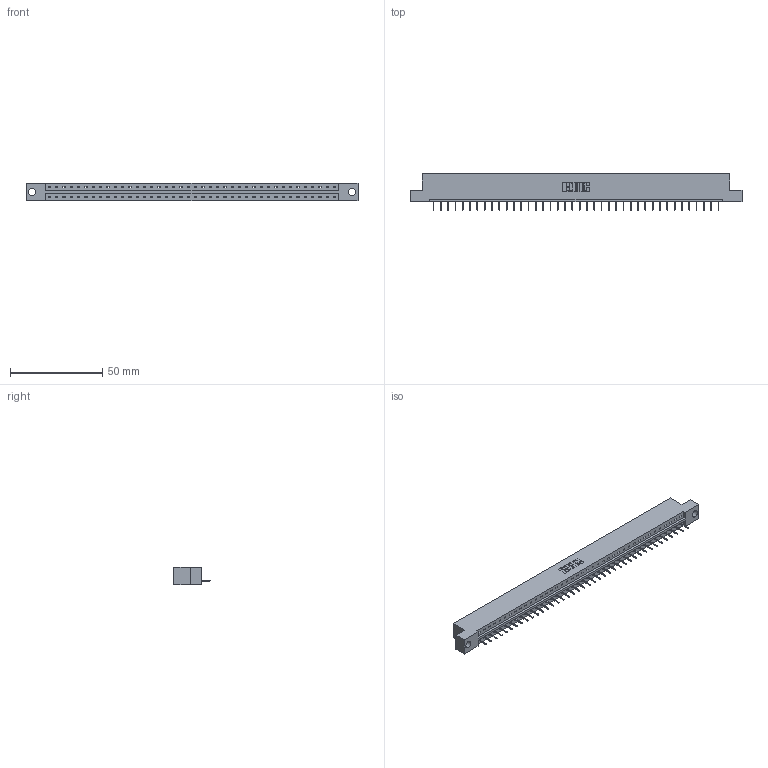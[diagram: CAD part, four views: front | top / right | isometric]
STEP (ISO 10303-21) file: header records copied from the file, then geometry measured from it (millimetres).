
FILE_DESCRIPTION (( 'STEP AP203' ), '1' );
FILE_NAME ('833-040-524-104.STEP', '2020-06-03T16:27:49', ( '' ), ( '' ), 'SwSTEP 2.0', 'SolidWorks 2020', '' );
FILE_SCHEMA (( 'CONFIG_CONTROL_DESIGN' ));
Length unit declared in the file: inch
Products named in the file (3): 833-040-524-104; 345-292-001_345-293-124; 833 Part_Flush - .156 Dia - TH
Assembly tree (41 placements, depth 2):
  833-040-524-104
    833 Part_Flush - .156 Dia - TH
    345-292-001_345-293-124  x40
Bounding box: 180.04 x 19.69 x 9.4 mm (x, y, z)
Volume: 17853.6 mm3; surface area: 18556.5 mm2
Topology: 41 solids, 41 shells, 2594 faces, 7511 edges, 4846 vertices
Faces by surface type: plane 1990, cylinder 604
Entity records: 24789 total; most frequent: CARTESIAN_POINT 4282, ORIENTED_EDGE 4258, DIRECTION 3617, EDGE_CURVE 2129, LINE 2005, VECTOR 2005, VERTEX_POINT 1414, AXIS2_PLACEMENT_3D 806
